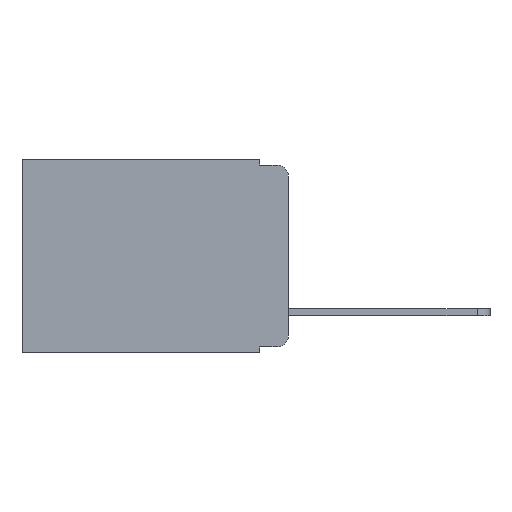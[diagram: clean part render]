
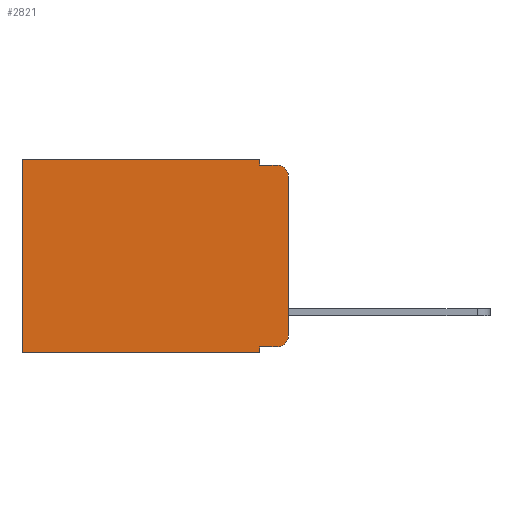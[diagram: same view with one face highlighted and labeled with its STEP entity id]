
A CAD part, left-side view. The second image highlights one B-rep face of the part: STEP entity #2821.
In plain terms, the highlighted planar face has unit normal (-1, 0, 0).
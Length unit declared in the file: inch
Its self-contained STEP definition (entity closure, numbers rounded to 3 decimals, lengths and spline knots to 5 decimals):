
#60 = ORIENTED_EDGE ( 'NONE', *, *, #17906, .F. ) ;
#127 = ORIENTED_EDGE ( 'NONE', *, *, #9748, .F. ) ;
#193 = ORIENTED_EDGE ( 'NONE', *, *, #8722, .T. ) ;
#324 = ORIENTED_EDGE ( 'NONE', *, *, #6723, .T. ) ;
#507 = EDGE_CURVE ( 'NONE', #11992, #11312, #12986, .T. ) ;
#621 = CARTESIAN_POINT ( 'NONE',  ( 0.298, 0., 0. ) ) ;
#748 = CARTESIAN_POINT ( 'NONE',  ( 0.298, 0.051, -0.333 ) ) ;
#804 = CARTESIAN_POINT ( 'NONE',  ( 0.298, 0.02, -0.333 ) ) ;
#1002 = DIRECTION ( 'NONE',  ( 0., 0., -1. ) ) ;
#1341 = EDGE_LOOP ( 'NONE', ( #60, #10763, #10279, #11140, #11341, #12119, #12415, #127, #193, #324 ) ) ;
#1442 = VECTOR ( 'NONE', #18955, 39.37008 ) ;
#1819 = VECTOR ( 'NONE', #13530, 39.37008 ) ;
#2707 = AXIS2_PLACEMENT_3D ( 'NONE', #19496, #10405, #1002 ) ;
#2821 = ADVANCED_FACE ( 'NONE', ( #15948 ), #14658, .F. ) ;
#2872 = CARTESIAN_POINT ( 'NONE',  ( 0.298, 0., 0. ) ) ;
#3626 = CARTESIAN_POINT ( 'NONE',  ( 0.298, 0., 0. ) ) ;
#3703 = VERTEX_POINT ( 'NONE', #12235 ) ;
#3993 = CARTESIAN_POINT ( 'NONE',  ( 0.298, 0.473, -0.343 ) ) ;
#4385 = LINE ( 'NONE', #13103, #16133 ) ;
#4485 = CARTESIAN_POINT ( 'NONE',  ( 0.298, 0., -0.343 ) ) ;
#5265 = CARTESIAN_POINT ( 'NONE',  ( 0.298, 0., -0.03 ) ) ;
#5640 = DIRECTION ( 'NONE',  ( 0., 1., 0. ) ) ;
#5813 = CARTESIAN_POINT ( 'NONE',  ( 0.298, 0.02, -0.01 ) ) ;
#6213 = EDGE_CURVE ( 'NONE', #3703, #15080, #10321, .T. ) ;
#6214 = VERTEX_POINT ( 'NONE', #16730 ) ;
#6647 = CARTESIAN_POINT ( 'NONE',  ( 0.298, 0.02, -0.03 ) ) ;
#6723 = EDGE_CURVE ( 'NONE', #18697, #6214, #10303, .T. ) ;
#6931 = LINE ( 'NONE', #16168, #14999 ) ;
#7445 = VECTOR ( 'NONE', #15952, 39.37008 ) ;
#7916 = LINE ( 'NONE', #14456, #7445 ) ;
#8050 = DIRECTION ( 'NONE',  ( 0., 0., -1. ) ) ;
#8163 = DIRECTION ( 'NONE',  ( 0., 0., -1. ) ) ;
#8196 = LINE ( 'NONE', #9630, #11318 ) ;
#8233 = VERTEX_POINT ( 'NONE', #5813 ) ;
#8588 = DIRECTION ( 'NONE',  ( 0., 0., -1. ) ) ;
#8722 = EDGE_CURVE ( 'NONE', #12568, #18697, #6931, .T. ) ;
#8778 = CARTESIAN_POINT ( 'NONE',  ( 0.298, 0.051, -0.343 ) ) ;
#8818 = AXIS2_PLACEMENT_3D ( 'NONE', #621, #17697, #8588 ) ;
#9630 = CARTESIAN_POINT ( 'NONE',  ( 0.298, 0.051, 0. ) ) ;
#9672 = LINE ( 'NONE', #10440, #1819 ) ;
#9748 = EDGE_CURVE ( 'NONE', #12568, #11992, #4385, .T. ) ;
#9800 = LINE ( 'NONE', #3626, #1442 ) ;
#9908 = CARTESIAN_POINT ( 'NONE',  ( 0.298, 0.051, -0.01 ) ) ;
#10199 = CARTESIAN_POINT ( 'NONE',  ( 0.298, 0.473, 0. ) ) ;
#10279 = ORIENTED_EDGE ( 'NONE', *, *, #13862, .F. ) ;
#10303 = CIRCLE ( 'NONE', #2707, 0.02 ) ;
#10321 = LINE ( 'NONE', #2872, #13914 ) ;
#10405 = DIRECTION ( 'NONE',  ( -1., 0., 0. ) ) ;
#10440 = CARTESIAN_POINT ( 'NONE',  ( 0.298, 0.473, 0. ) ) ;
#10763 = ORIENTED_EDGE ( 'NONE', *, *, #14854, .T. ) ;
#10784 = EDGE_CURVE ( 'NONE', #15080, #11312, #9672, .T. ) ;
#11140 = ORIENTED_EDGE ( 'NONE', *, *, #12836, .F. ) ;
#11312 = VERTEX_POINT ( 'NONE', #3993 ) ;
#11318 = VECTOR ( 'NONE', #8050, 39.37008 ) ;
#11341 = ORIENTED_EDGE ( 'NONE', *, *, #6213, .T. ) ;
#11992 = VERTEX_POINT ( 'NONE', #8778 ) ;
#12119 = ORIENTED_EDGE ( 'NONE', *, *, #10784, .T. ) ;
#12235 = CARTESIAN_POINT ( 'NONE',  ( 0.298, 0.051, 0. ) ) ;
#12415 = ORIENTED_EDGE ( 'NONE', *, *, #507, .F. ) ;
#12452 = VERTEX_POINT ( 'NONE', #9908 ) ;
#12568 = VERTEX_POINT ( 'NONE', #748 ) ;
#12836 = EDGE_CURVE ( 'NONE', #3703, #12452, #8196, .T. ) ;
#12986 = LINE ( 'NONE', #4485, #16040 ) ;
#13103 = CARTESIAN_POINT ( 'NONE',  ( 0.298, 0.051, 0. ) ) ;
#13125 = CIRCLE ( 'NONE', #20035, 0.02 ) ;
#13530 = DIRECTION ( 'NONE',  ( 0., 0., -1. ) ) ;
#13862 = EDGE_CURVE ( 'NONE', #12452, #8233, #7916, .T. ) ;
#13914 = VECTOR ( 'NONE', #15222, 39.37008 ) ;
#14456 = CARTESIAN_POINT ( 'NONE',  ( 0.298, 0.051, -0.01 ) ) ;
#14620 = DIRECTION ( 'NONE',  ( 0., 0., -1. ) ) ;
#14658 = PLANE ( 'NONE',  #8818 ) ;
#14854 = EDGE_CURVE ( 'NONE', #16202, #8233, #13125, .T. ) ;
#14999 = VECTOR ( 'NONE', #19219, 39.37008 ) ;
#15080 = VERTEX_POINT ( 'NONE', #10199 ) ;
#15222 = DIRECTION ( 'NONE',  ( 0., 1., 0. ) ) ;
#15948 = FACE_OUTER_BOUND ( 'NONE', #1341, .T. ) ;
#15952 = DIRECTION ( 'NONE',  ( 0., -1., 0. ) ) ;
#16040 = VECTOR ( 'NONE', #5640, 39.37008 ) ;
#16133 = VECTOR ( 'NONE', #14620, 39.37008 ) ;
#16168 = CARTESIAN_POINT ( 'NONE',  ( 0.298, 0.051, -0.333 ) ) ;
#16202 = VERTEX_POINT ( 'NONE', #5265 ) ;
#16730 = CARTESIAN_POINT ( 'NONE',  ( 0.298, 0., -0.313 ) ) ;
#17262 = DIRECTION ( 'NONE',  ( -1., 0., 0. ) ) ;
#17697 = DIRECTION ( 'NONE',  ( 1., 0., 0. ) ) ;
#17906 = EDGE_CURVE ( 'NONE', #16202, #6214, #9800, .T. ) ;
#18697 = VERTEX_POINT ( 'NONE', #804 ) ;
#18955 = DIRECTION ( 'NONE',  ( 0., 0., -1. ) ) ;
#19219 = DIRECTION ( 'NONE',  ( 0., -1., 0. ) ) ;
#19496 = CARTESIAN_POINT ( 'NONE',  ( 0.298, 0.02, -0.313 ) ) ;
#20035 = AXIS2_PLACEMENT_3D ( 'NONE', #6647, #17262, #8163 ) ;
